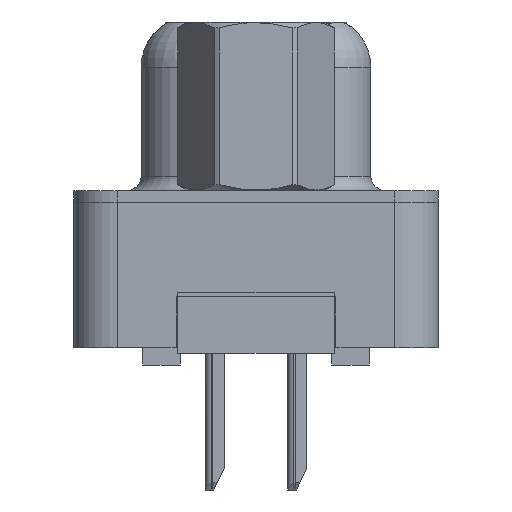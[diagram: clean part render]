
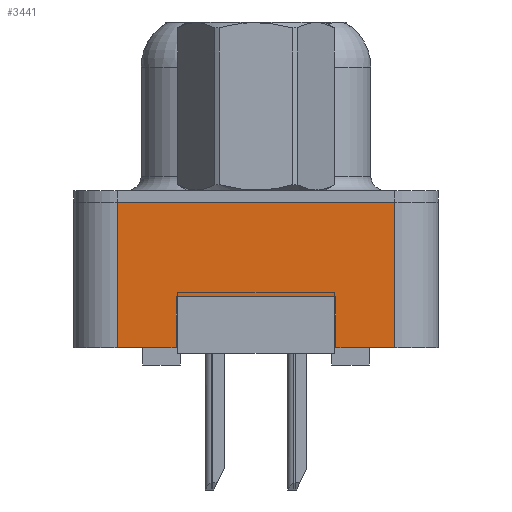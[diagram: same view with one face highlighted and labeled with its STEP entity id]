
A CAD part, left-side view. The second image highlights one B-rep face of the part: STEP entity #3441.
In plain terms, the highlighted planar face has unit normal (-1, 0, 0).
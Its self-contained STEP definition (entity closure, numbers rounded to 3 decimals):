
#203 = CARTESIAN_POINT ( 'NONE',  ( -2.91, -4.775, -5. ) ) ;
#781 = LINE ( 'NONE', #3371, #14362 ) ;
#808 = CARTESIAN_POINT ( 'NONE',  ( -2.91, 4.775, -5. ) ) ;
#830 = VECTOR ( 'NONE', #7279, 1000. ) ;
#2006 = VERTEX_POINT ( 'NONE', #3422 ) ;
#2448 = CARTESIAN_POINT ( 'NONE',  ( -2.91, -4.775, -5. ) ) ;
#2450 = LINE ( 'NONE', #11249, #7985 ) ;
#2469 = VERTEX_POINT ( 'NONE', #14618 ) ;
#2589 = LINE ( 'NONE', #2448, #13818 ) ;
#2719 = CARTESIAN_POINT ( 'NONE',  ( -2.91, 2.75, -3.25 ) ) ;
#3272 = VERTEX_POINT ( 'NONE', #27616 ) ;
#3371 = CARTESIAN_POINT ( 'NONE',  ( -2.91, -4.775, -5. ) ) ;
#3422 = CARTESIAN_POINT ( 'NONE',  ( -2.91, 2.75, -5. ) ) ;
#3441 = ADVANCED_FACE ( 'NONE', ( #4799 ), #22925, .T. ) ;
#4629 = ORIENTED_EDGE ( 'NONE', *, *, #11561, .T. ) ;
#4799 = FACE_OUTER_BOUND ( 'NONE', #27901, .T. ) ;
#4914 = DIRECTION ( 'NONE',  ( 0., 0., -1. ) ) ;
#5122 = LINE ( 'NONE', #808, #830 ) ;
#5200 = CARTESIAN_POINT ( 'NONE',  ( -2.91, -4.775, -5. ) ) ;
#5377 = EDGE_CURVE ( 'NONE', #9298, #20907, #18553, .T. ) ;
#6295 = VECTOR ( 'NONE', #27769, 1000. ) ;
#6520 = CARTESIAN_POINT ( 'NONE',  ( -2.91, -2.75, -3.25 ) ) ;
#6751 = ORIENTED_EDGE ( 'NONE', *, *, #9151, .F. ) ;
#7175 = DIRECTION ( 'NONE',  ( 0., 1., 0. ) ) ;
#7279 = DIRECTION ( 'NONE',  ( 0., 0., 1. ) ) ;
#7985 = VECTOR ( 'NONE', #7175, 1000. ) ;
#8408 = AXIS2_PLACEMENT_3D ( 'NONE', #11468, #13620, #22496 ) ;
#8713 = ORIENTED_EDGE ( 'NONE', *, *, #5377, .T. ) ;
#9151 = EDGE_CURVE ( 'NONE', #3272, #13718, #24075, .T. ) ;
#9237 = ORIENTED_EDGE ( 'NONE', *, *, #23820, .F. ) ;
#9267 = CARTESIAN_POINT ( 'NONE',  ( -2.91, -2.75, -5. ) ) ;
#9298 = VERTEX_POINT ( 'NONE', #9267 ) ;
#9409 = VERTEX_POINT ( 'NONE', #6520 ) ;
#10599 = EDGE_CURVE ( 'NONE', #2469, #3272, #5122, .T. ) ;
#11249 = CARTESIAN_POINT ( 'NONE',  ( -2.91, 2.75, -3.25 ) ) ;
#11468 = CARTESIAN_POINT ( 'NONE',  ( -2.91, -4.775, -5. ) ) ;
#11561 = EDGE_CURVE ( 'NONE', #2469, #2006, #2589, .T. ) ;
#13294 = ORIENTED_EDGE ( 'NONE', *, *, #21124, .T. ) ;
#13534 = LINE ( 'NONE', #2719, #6295 ) ;
#13620 = DIRECTION ( 'NONE',  ( -1., 0., 0. ) ) ;
#13626 = CARTESIAN_POINT ( 'NONE',  ( -2.91, 2.75, -3.25 ) ) ;
#13718 = VERTEX_POINT ( 'NONE', #14423 ) ;
#13739 = DIRECTION ( 'NONE',  ( 0., -1., 0. ) ) ;
#13818 = VECTOR ( 'NONE', #18360, 1000. ) ;
#14362 = VECTOR ( 'NONE', #25532, 1000. ) ;
#14423 = CARTESIAN_POINT ( 'NONE',  ( -2.91, -4.775, 0. ) ) ;
#14618 = CARTESIAN_POINT ( 'NONE',  ( -2.91, 4.775, -5. ) ) ;
#15433 = VECTOR ( 'NONE', #13739, 1000. ) ;
#16288 = ORIENTED_EDGE ( 'NONE', *, *, #16582, .F. ) ;
#16582 = EDGE_CURVE ( 'NONE', #26151, #2006, #13534, .T. ) ;
#18360 = DIRECTION ( 'NONE',  ( 0., -1., 0. ) ) ;
#18546 = CARTESIAN_POINT ( 'NONE',  ( -2.91, -2.75, -3.25 ) ) ;
#18553 = LINE ( 'NONE', #5200, #15433 ) ;
#19455 = EDGE_CURVE ( 'NONE', #9409, #9298, #25066, .T. ) ;
#20519 = ORIENTED_EDGE ( 'NONE', *, *, #10599, .F. ) ;
#20907 = VERTEX_POINT ( 'NONE', #203 ) ;
#21124 = EDGE_CURVE ( 'NONE', #20907, #13718, #781, .T. ) ;
#21758 = DIRECTION ( 'NONE',  ( 0., -1., 0. ) ) ;
#22048 = VECTOR ( 'NONE', #21758, 1000. ) ;
#22496 = DIRECTION ( 'NONE',  ( 0., 0., 1. ) ) ;
#22925 = PLANE ( 'NONE',  #8408 ) ;
#22975 = ORIENTED_EDGE ( 'NONE', *, *, #19455, .T. ) ;
#23820 = EDGE_CURVE ( 'NONE', #9409, #26151, #2450, .T. ) ;
#24037 = VECTOR ( 'NONE', #4914, 1000. ) ;
#24075 = LINE ( 'NONE', #26267, #22048 ) ;
#25066 = LINE ( 'NONE', #18546, #24037 ) ;
#25532 = DIRECTION ( 'NONE',  ( 0., 0., 1. ) ) ;
#26151 = VERTEX_POINT ( 'NONE', #13626 ) ;
#26267 = CARTESIAN_POINT ( 'NONE',  ( -2.91, -4.775, 0. ) ) ;
#27616 = CARTESIAN_POINT ( 'NONE',  ( -2.91, 4.775, 0. ) ) ;
#27769 = DIRECTION ( 'NONE',  ( 0., 0., -1. ) ) ;
#27901 = EDGE_LOOP ( 'NONE', ( #22975, #8713, #13294, #6751, #20519, #4629, #16288, #9237 ) ) ;
